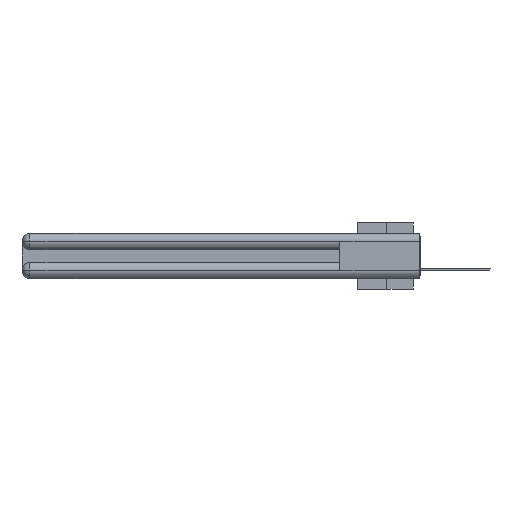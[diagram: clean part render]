
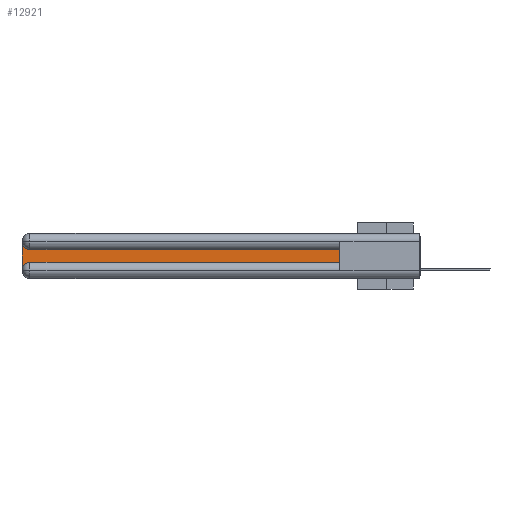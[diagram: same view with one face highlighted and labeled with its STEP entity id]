
A CAD part, left-side view. The second image highlights one B-rep face of the part: STEP entity #12921.
In plain terms, the highlighted planar face has unit normal (-1, 0, 0).
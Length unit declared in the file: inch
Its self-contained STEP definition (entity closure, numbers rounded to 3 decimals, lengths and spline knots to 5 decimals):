
#782 = VERTEX_POINT ( 'NONE', #950 ) ;
#950 = CARTESIAN_POINT ( 'NONE',  ( 0.075, 2.94, -0.1225 ) ) ;
#1155 = EDGE_CURVE ( 'NONE', #29546, #782, #22778, .T. ) ;
#1540 = VERTEX_POINT ( 'NONE', #11024 ) ;
#1567 = VERTEX_POINT ( 'NONE', #22219 ) ;
#1632 = AXIS2_PLACEMENT_3D ( 'NONE', #8529, #33248, #33020 ) ;
#2640 = ORIENTED_EDGE ( 'NONE', *, *, #20815, .T. ) ;
#3958 = ORIENTED_EDGE ( 'NONE', *, *, #1155, .T. ) ;
#5538 = ORIENTED_EDGE ( 'NONE', *, *, #25681, .T. ) ;
#6065 = DIRECTION ( 'NONE',  ( 0., 0., -1. ) ) ;
#6736 = CARTESIAN_POINT ( 'NONE',  ( 0.075, 3., -0.2175 ) ) ;
#7334 = VECTOR ( 'NONE', #12523, 39.37008 ) ;
#7707 = PLANE ( 'NONE',  #11791 ) ;
#7839 = DIRECTION ( 'NONE',  ( 0., 0., 1. ) ) ;
#8093 = DIRECTION ( 'NONE',  ( 0., -1., 0. ) ) ;
#8529 = CARTESIAN_POINT ( 'NONE',  ( 0.075, 2.94, -0.0625 ) ) ;
#9894 = ORIENTED_EDGE ( 'NONE', *, *, #33456, .T. ) ;
#11024 = CARTESIAN_POINT ( 'NONE',  ( 0.075, 3., -0.2775 ) ) ;
#11791 = AXIS2_PLACEMENT_3D ( 'NONE', #31144, #33767, #6065 ) ;
#11904 = DIRECTION ( 'NONE',  ( 0., 0., -1. ) ) ;
#12523 = DIRECTION ( 'NONE',  ( 0., 1., 0. ) ) ;
#12710 = LINE ( 'NONE', #32530, #35153 ) ;
#12921 = ADVANCED_FACE ( 'NONE', ( #17914 ), #7707, .F. ) ;
#13637 = CARTESIAN_POINT ( 'NONE',  ( 0.075, 3., -0.0625 ) ) ;
#13795 = AXIS2_PLACEMENT_3D ( 'NONE', #21069, #32271, #15760 ) ;
#14111 = CARTESIAN_POINT ( 'NONE',  ( 0.075, 0.6, -0.1225 ) ) ;
#15244 = VERTEX_POINT ( 'NONE', #13637 ) ;
#15315 = CIRCLE ( 'NONE', #13795, 0.06 ) ;
#15760 = DIRECTION ( 'NONE',  ( 0., 0., -1. ) ) ;
#15811 = ORIENTED_EDGE ( 'NONE', *, *, #20076, .T. ) ;
#16148 = CARTESIAN_POINT ( 'NONE',  ( 0.075, 0.6, -0.2175 ) ) ;
#17914 = FACE_OUTER_BOUND ( 'NONE', #30577, .T. ) ;
#20076 = EDGE_CURVE ( 'NONE', #15244, #1540, #28292, .T. ) ;
#20763 = VERTEX_POINT ( 'NONE', #31920 ) ;
#20815 = EDGE_CURVE ( 'NONE', #1540, #20763, #15315, .T. ) ;
#21069 = CARTESIAN_POINT ( 'NONE',  ( 0.075, 2.94, -0.2775 ) ) ;
#22219 = CARTESIAN_POINT ( 'NONE',  ( 0.075, 0.6, -0.2175 ) ) ;
#22778 = LINE ( 'NONE', #34726, #7334 ) ;
#25681 = EDGE_CURVE ( 'NONE', #1567, #29546, #12710, .T. ) ;
#27598 = CIRCLE ( 'NONE', #1632, 0.06 ) ;
#27833 = VECTOR ( 'NONE', #11904, 39.37008 ) ;
#28292 = LINE ( 'NONE', #6736, #27833 ) ;
#29546 = VERTEX_POINT ( 'NONE', #14111 ) ;
#29556 = LINE ( 'NONE', #16148, #35600 ) ;
#30577 = EDGE_LOOP ( 'NONE', ( #3958, #35612, #15811, #2640, #9894, #5538 ) ) ;
#31144 = CARTESIAN_POINT ( 'NONE',  ( 0.075, 3., -0.1225 ) ) ;
#31920 = CARTESIAN_POINT ( 'NONE',  ( 0.075, 2.94, -0.2175 ) ) ;
#32271 = DIRECTION ( 'NONE',  ( 1., 0., 0. ) ) ;
#32530 = CARTESIAN_POINT ( 'NONE',  ( 0.075, 0.6, -0.2175 ) ) ;
#33020 = DIRECTION ( 'NONE',  ( 0., 0., -1. ) ) ;
#33248 = DIRECTION ( 'NONE',  ( 1., 0., 0. ) ) ;
#33456 = EDGE_CURVE ( 'NONE', #20763, #1567, #29556, .T. ) ;
#33767 = DIRECTION ( 'NONE',  ( 1., 0., 0. ) ) ;
#34726 = CARTESIAN_POINT ( 'NONE',  ( 0.075, 0.6, -0.1225 ) ) ;
#35153 = VECTOR ( 'NONE', #7839, 39.37008 ) ;
#35531 = EDGE_CURVE ( 'NONE', #782, #15244, #27598, .T. ) ;
#35600 = VECTOR ( 'NONE', #8093, 39.37008 ) ;
#35612 = ORIENTED_EDGE ( 'NONE', *, *, #35531, .T. ) ;
